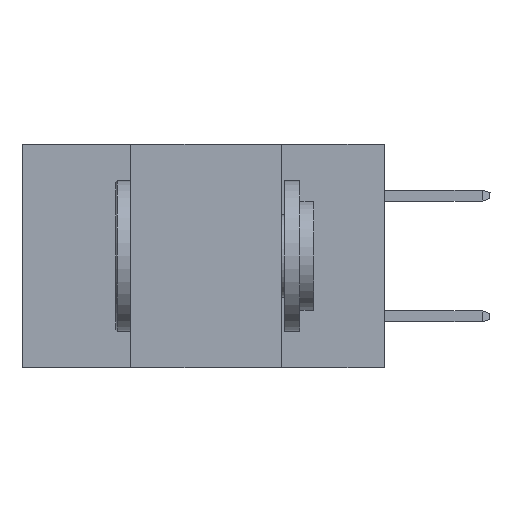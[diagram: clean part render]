
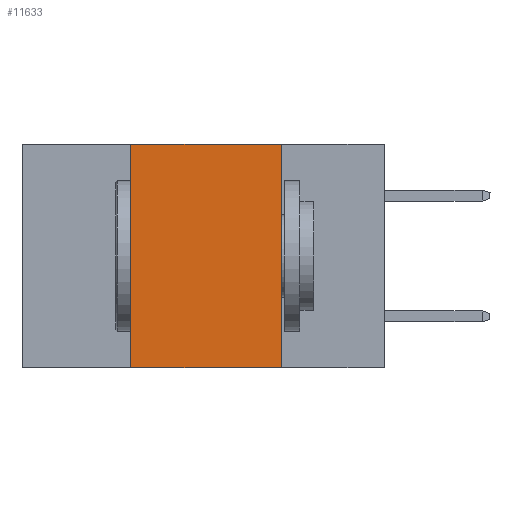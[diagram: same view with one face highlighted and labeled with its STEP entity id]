
A CAD part, left-side view. The second image highlights one B-rep face of the part: STEP entity #11633.
In plain terms, the highlighted planar face has unit normal (-1, 0, 0).
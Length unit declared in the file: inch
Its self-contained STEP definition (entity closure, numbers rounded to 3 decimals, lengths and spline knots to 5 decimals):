
#150 = CARTESIAN_POINT ( 'NONE',  ( 0., 0.42, 0. ) ) ;
#208 = AXIS2_PLACEMENT_3D ( 'NONE', #10874, #4157, #4006 ) ;
#1745 = VECTOR ( 'NONE', #11321, 39.37008 ) ;
#1922 = VERTEX_POINT ( 'NONE', #2387 ) ;
#2387 = CARTESIAN_POINT ( 'NONE',  ( 0., 0.17, 0. ) ) ;
#2914 = LINE ( 'NONE', #19645, #11384 ) ;
#3108 = ORIENTED_EDGE ( 'NONE', *, *, #10949, .F. ) ;
#3442 = DIRECTION ( 'NONE',  ( 0., 0., 1. ) ) ;
#3523 = VERTEX_POINT ( 'NONE', #8149 ) ;
#4006 = DIRECTION ( 'NONE',  ( 0., 0., -1. ) ) ;
#4157 = DIRECTION ( 'NONE',  ( 1., 0., 0. ) ) ;
#4403 = EDGE_LOOP ( 'NONE', ( #3108, #11672, #12801, #17342 ) ) ;
#5719 = VERTEX_POINT ( 'NONE', #12393 ) ;
#7909 = EDGE_CURVE ( 'NONE', #3523, #1922, #8090, .T. ) ;
#8090 = LINE ( 'NONE', #21013, #12634 ) ;
#8149 = CARTESIAN_POINT ( 'NONE',  ( 0., 0.42, 0. ) ) ;
#8459 = EDGE_CURVE ( 'NONE', #18586, #5719, #11289, .T. ) ;
#9236 = DIRECTION ( 'NONE',  ( 0., -1., 0. ) ) ;
#9272 = FACE_OUTER_BOUND ( 'NONE', #4403, .T. ) ;
#10731 = PLANE ( 'NONE',  #208 ) ;
#10874 = CARTESIAN_POINT ( 'NONE',  ( 0., 0.6, 0. ) ) ;
#10949 = EDGE_CURVE ( 'NONE', #1922, #5719, #2914, .T. ) ;
#11289 = LINE ( 'NONE', #13012, #1745 ) ;
#11321 = DIRECTION ( 'NONE',  ( 0., -1., 0. ) ) ;
#11384 = VECTOR ( 'NONE', #21240, 39.37008 ) ;
#11633 = ADVANCED_FACE ( 'NONE', ( #9272 ), #10731, .F. ) ;
#11672 = ORIENTED_EDGE ( 'NONE', *, *, #7909, .F. ) ;
#12393 = CARTESIAN_POINT ( 'NONE',  ( 0., 0.17, -0.37 ) ) ;
#12634 = VECTOR ( 'NONE', #9236, 39.37008 ) ;
#12801 = ORIENTED_EDGE ( 'NONE', *, *, #19325, .F. ) ;
#13012 = CARTESIAN_POINT ( 'NONE',  ( 0., 0.6, -0.37 ) ) ;
#15102 = VECTOR ( 'NONE', #3442, 39.37008 ) ;
#16939 = LINE ( 'NONE', #150, #15102 ) ;
#17342 = ORIENTED_EDGE ( 'NONE', *, *, #8459, .T. ) ;
#18586 = VERTEX_POINT ( 'NONE', #21348 ) ;
#19325 = EDGE_CURVE ( 'NONE', #18586, #3523, #16939, .T. ) ;
#19645 = CARTESIAN_POINT ( 'NONE',  ( 0., 0.17, 0. ) ) ;
#21013 = CARTESIAN_POINT ( 'NONE',  ( 0., 0.6, 0. ) ) ;
#21240 = DIRECTION ( 'NONE',  ( 0., 0., -1. ) ) ;
#21348 = CARTESIAN_POINT ( 'NONE',  ( 0., 0.42, -0.37 ) ) ;
